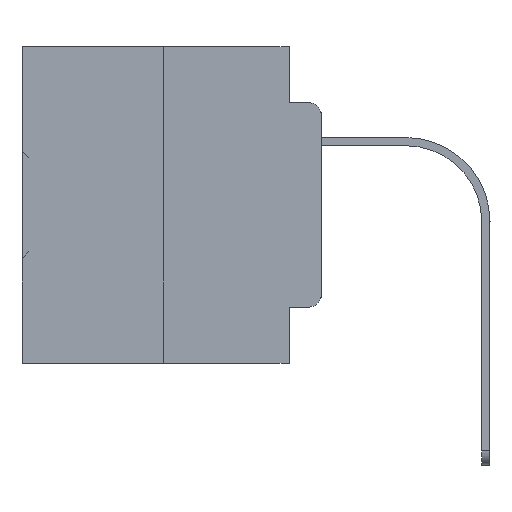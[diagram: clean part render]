
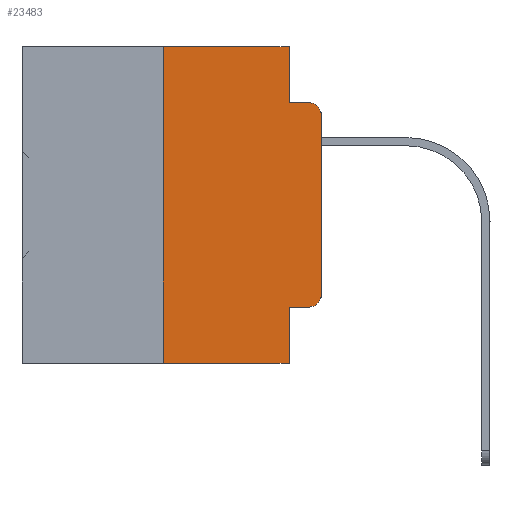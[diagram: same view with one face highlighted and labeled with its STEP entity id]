
A CAD part, left-side view. The second image highlights one B-rep face of the part: STEP entity #23483.
In plain terms, the highlighted planar face has unit normal (-1, 0, 0).
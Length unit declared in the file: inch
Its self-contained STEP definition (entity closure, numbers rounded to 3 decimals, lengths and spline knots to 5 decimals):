
#950 = LINE ( 'NONE', #7214, #20643 ) ;
#1110 = ORIENTED_EDGE ( 'NONE', *, *, #20276, .T. ) ;
#1693 = CARTESIAN_POINT ( 'NONE',  ( 0., 0.051, 0. ) ) ;
#2436 = ORIENTED_EDGE ( 'NONE', *, *, #33368, .F. ) ;
#2475 = ORIENTED_EDGE ( 'NONE', *, *, #4451, .T. ) ;
#2977 = EDGE_CURVE ( 'NONE', #3856, #14477, #20201, .T. ) ;
#3204 = AXIS2_PLACEMENT_3D ( 'NONE', #21176, #21740, #4642 ) ;
#3236 = LINE ( 'NONE', #15014, #13907 ) ;
#3405 = VERTEX_POINT ( 'NONE', #36887 ) ;
#3431 = LINE ( 'NONE', #11994, #11917 ) ;
#3856 = VERTEX_POINT ( 'NONE', #35086 ) ;
#4323 = DIRECTION ( 'NONE',  ( -1., 0., 0. ) ) ;
#4451 = EDGE_CURVE ( 'NONE', #3405, #29163, #8119, .T. ) ;
#4642 = DIRECTION ( 'NONE',  ( 0., 0., -1. ) ) ;
#4990 = VERTEX_POINT ( 'NONE', #5246 ) ;
#4994 = CARTESIAN_POINT ( 'NONE',  ( 0., 0.051, -0.0885 ) ) ;
#5246 = CARTESIAN_POINT ( 'NONE',  ( 0., 0., -0.1085 ) ) ;
#7066 = LINE ( 'NONE', #24351, #25478 ) ;
#7214 = CARTESIAN_POINT ( 'NONE',  ( 0., 0.25, 0. ) ) ;
#8119 = CIRCLE ( 'NONE', #28143, 0.02 ) ;
#8569 = VECTOR ( 'NONE', #11672, 39.37008 ) ;
#8749 = DIRECTION ( 'NONE',  ( 0., -1., 0. ) ) ;
#9386 = ORIENTED_EDGE ( 'NONE', *, *, #18793, .F. ) ;
#10933 = EDGE_CURVE ( 'NONE', #4990, #22416, #28327, .T. ) ;
#11092 = CARTESIAN_POINT ( 'NONE',  ( 0., 0., -0.3915 ) ) ;
#11672 = DIRECTION ( 'NONE',  ( 0., 0., -1. ) ) ;
#11917 = VECTOR ( 'NONE', #35947, 39.37008 ) ;
#11994 = CARTESIAN_POINT ( 'NONE',  ( 0., 0.051, -0.0885 ) ) ;
#12052 = ORIENTED_EDGE ( 'NONE', *, *, #26480, .F. ) ;
#12511 = ORIENTED_EDGE ( 'NONE', *, *, #2977, .F. ) ;
#12723 = CARTESIAN_POINT ( 'NONE',  ( 0., 0.02, -0.3915 ) ) ;
#12839 = VECTOR ( 'NONE', #30104, 39.37008 ) ;
#12938 = CARTESIAN_POINT ( 'NONE',  ( 0., 0.051, 0. ) ) ;
#13381 = PLANE ( 'NONE',  #3204 ) ;
#13907 = VECTOR ( 'NONE', #8749, 39.37008 ) ;
#14450 = ORIENTED_EDGE ( 'NONE', *, *, #10933, .T. ) ;
#14477 = VERTEX_POINT ( 'NONE', #19150 ) ;
#14620 = EDGE_LOOP ( 'NONE', ( #27715, #14450, #12052, #2436, #9386, #20859, #31962, #12511, #1110, #2475 ) ) ;
#14984 = AXIS2_PLACEMENT_3D ( 'NONE', #25016, #4323, #36285 ) ;
#15014 = CARTESIAN_POINT ( 'NONE',  ( 0., 0.473, -0.5 ) ) ;
#15287 = VERTEX_POINT ( 'NONE', #12938 ) ;
#16141 = LINE ( 'NONE', #1693, #21053 ) ;
#16319 = VERTEX_POINT ( 'NONE', #27011 ) ;
#17389 = CARTESIAN_POINT ( 'NONE',  ( 0., 0., 0. ) ) ;
#17865 = EDGE_CURVE ( 'NONE', #17903, #14477, #3236, .T. ) ;
#17903 = VERTEX_POINT ( 'NONE', #32132 ) ;
#18793 = EDGE_CURVE ( 'NONE', #16319, #15287, #7066, .T. ) ;
#19150 = CARTESIAN_POINT ( 'NONE',  ( 0., 0.051, -0.5 ) ) ;
#19197 = EDGE_CURVE ( 'NONE', #17903, #16319, #950, .T. ) ;
#20201 = LINE ( 'NONE', #31429, #8569 ) ;
#20276 = EDGE_CURVE ( 'NONE', #3856, #3405, #20976, .T. ) ;
#20643 = VECTOR ( 'NONE', #27359, 39.37008 ) ;
#20859 = ORIENTED_EDGE ( 'NONE', *, *, #19197, .F. ) ;
#20976 = LINE ( 'NONE', #21161, #12839 ) ;
#21053 = VECTOR ( 'NONE', #24861, 39.37008 ) ;
#21161 = CARTESIAN_POINT ( 'NONE',  ( 0., 0.051, -0.4115 ) ) ;
#21176 = CARTESIAN_POINT ( 'NONE',  ( 0., 0.473, 0. ) ) ;
#21740 = DIRECTION ( 'NONE',  ( 1., 0., 0. ) ) ;
#22075 = VECTOR ( 'NONE', #32400, 39.37008 ) ;
#22416 = VERTEX_POINT ( 'NONE', #28707 ) ;
#23483 = ADVANCED_FACE ( 'NONE', ( #27825 ), #13381, .F. ) ;
#24303 = DIRECTION ( 'NONE',  ( -1., 0., 0. ) ) ;
#24351 = CARTESIAN_POINT ( 'NONE',  ( 0., 0.473, 0. ) ) ;
#24861 = DIRECTION ( 'NONE',  ( 0., 0., -1. ) ) ;
#25016 = CARTESIAN_POINT ( 'NONE',  ( 0., 0.02, -0.1085 ) ) ;
#25478 = VECTOR ( 'NONE', #32936, 39.37008 ) ;
#26480 = EDGE_CURVE ( 'NONE', #27948, #22416, #3431, .T. ) ;
#27011 = CARTESIAN_POINT ( 'NONE',  ( 0., 0.25, 0. ) ) ;
#27359 = DIRECTION ( 'NONE',  ( 0., 0., 1. ) ) ;
#27715 = ORIENTED_EDGE ( 'NONE', *, *, #28902, .T. ) ;
#27825 = FACE_OUTER_BOUND ( 'NONE', #14620, .T. ) ;
#27948 = VERTEX_POINT ( 'NONE', #4994 ) ;
#28143 = AXIS2_PLACEMENT_3D ( 'NONE', #12723, #24303, #35936 ) ;
#28327 = CIRCLE ( 'NONE', #14984, 0.02 ) ;
#28707 = CARTESIAN_POINT ( 'NONE',  ( 0., 0.02, -0.0885 ) ) ;
#28902 = EDGE_CURVE ( 'NONE', #29163, #4990, #31649, .T. ) ;
#29163 = VERTEX_POINT ( 'NONE', #11092 ) ;
#30104 = DIRECTION ( 'NONE',  ( 0., -1., 0. ) ) ;
#31429 = CARTESIAN_POINT ( 'NONE',  ( 0., 0.051, 0. ) ) ;
#31649 = LINE ( 'NONE', #17389, #22075 ) ;
#31962 = ORIENTED_EDGE ( 'NONE', *, *, #17865, .T. ) ;
#32132 = CARTESIAN_POINT ( 'NONE',  ( 0., 0.25, -0.5 ) ) ;
#32400 = DIRECTION ( 'NONE',  ( 0., 0., 1. ) ) ;
#32936 = DIRECTION ( 'NONE',  ( 0., -1., 0. ) ) ;
#33368 = EDGE_CURVE ( 'NONE', #15287, #27948, #16141, .T. ) ;
#35086 = CARTESIAN_POINT ( 'NONE',  ( 0., 0.051, -0.4115 ) ) ;
#35936 = DIRECTION ( 'NONE',  ( 0., 0., -1. ) ) ;
#35947 = DIRECTION ( 'NONE',  ( 0., -1., 0. ) ) ;
#36285 = DIRECTION ( 'NONE',  ( 0., 0., -1. ) ) ;
#36887 = CARTESIAN_POINT ( 'NONE',  ( 0., 0.02, -0.4115 ) ) ;
